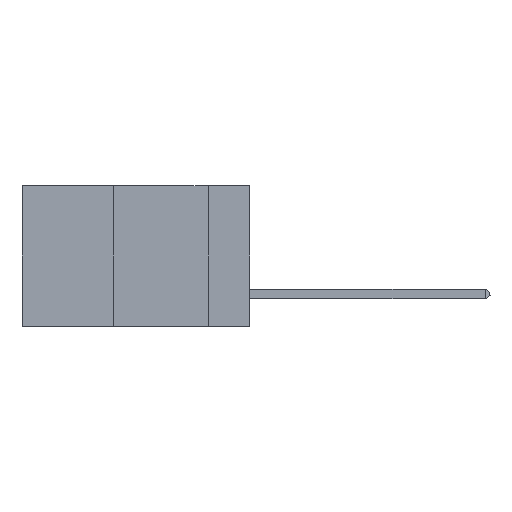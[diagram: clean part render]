
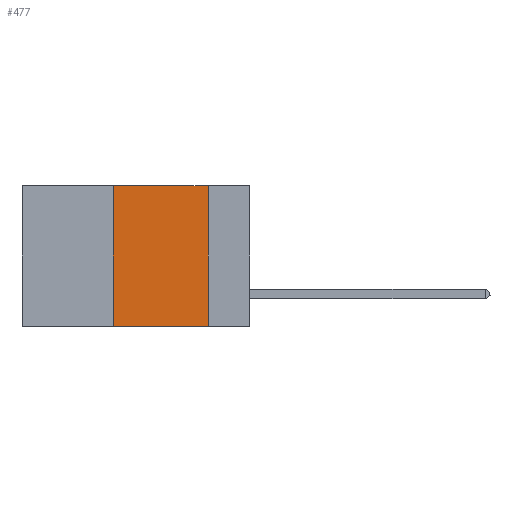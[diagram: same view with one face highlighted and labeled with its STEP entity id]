
A CAD part, left-side view. The second image highlights one B-rep face of the part: STEP entity #477.
In plain terms, the highlighted planar face has unit normal (-1, 0, 0).
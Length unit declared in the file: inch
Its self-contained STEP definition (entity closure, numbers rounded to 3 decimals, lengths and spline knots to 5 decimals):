
#151 = ORIENTED_EDGE ( 'NONE', *, *, #31321, .F. ) ;
#477 = ADVANCED_FACE ( 'NONE', ( #30734 ), #1263, .F. ) ;
#1263 = PLANE ( 'NONE',  #20618 ) ;
#2311 = LINE ( 'NONE', #8115, #15526 ) ;
#4240 = DIRECTION ( 'NONE',  ( 1., 0., 0. ) ) ;
#8035 = CARTESIAN_POINT ( 'NONE',  ( 0., 0.11, -0.37 ) ) ;
#8115 = CARTESIAN_POINT ( 'NONE',  ( 0., 0.36, 0. ) ) ;
#9543 = CARTESIAN_POINT ( 'NONE',  ( 0., 0.6, -0.37 ) ) ;
#12318 = CARTESIAN_POINT ( 'NONE',  ( 0., 0.6, 0. ) ) ;
#12811 = VERTEX_POINT ( 'NONE', #23126 ) ;
#14838 = LINE ( 'NONE', #23871, #15666 ) ;
#15526 = VECTOR ( 'NONE', #27342, 39.37008 ) ;
#15666 = VECTOR ( 'NONE', #31942, 39.37008 ) ;
#16629 = ORIENTED_EDGE ( 'NONE', *, *, #32675, .T. ) ;
#18580 = CARTESIAN_POINT ( 'NONE',  ( 0., 0.36, -0.37 ) ) ;
#20011 = EDGE_CURVE ( 'NONE', #21207, #20627, #14838, .T. ) ;
#20078 = CARTESIAN_POINT ( 'NONE',  ( 0., 0.6, 0. ) ) ;
#20618 = AXIS2_PLACEMENT_3D ( 'NONE', #12318, #4240, #30980 ) ;
#20627 = VERTEX_POINT ( 'NONE', #8035 ) ;
#21176 = DIRECTION ( 'NONE',  ( 0., -1., 0. ) ) ;
#21207 = VERTEX_POINT ( 'NONE', #27738 ) ;
#21573 = VECTOR ( 'NONE', #30868, 39.37008 ) ;
#22081 = EDGE_CURVE ( 'NONE', #12811, #21207, #25952, .T. ) ;
#23126 = CARTESIAN_POINT ( 'NONE',  ( 0., 0.36, 0. ) ) ;
#23871 = CARTESIAN_POINT ( 'NONE',  ( 0., 0.11, 0. ) ) ;
#25526 = VECTOR ( 'NONE', #21176, 39.37008 ) ;
#25952 = LINE ( 'NONE', #20078, #25526 ) ;
#27342 = DIRECTION ( 'NONE',  ( 0., 0., 1. ) ) ;
#27738 = CARTESIAN_POINT ( 'NONE',  ( 0., 0.11, 0. ) ) ;
#27911 = ORIENTED_EDGE ( 'NONE', *, *, #20011, .F. ) ;
#30734 = FACE_OUTER_BOUND ( 'NONE', #32633, .T. ) ;
#30868 = DIRECTION ( 'NONE',  ( 0., -1., 0. ) ) ;
#30980 = DIRECTION ( 'NONE',  ( 0., 0., -1. ) ) ;
#31321 = EDGE_CURVE ( 'NONE', #32310, #12811, #2311, .T. ) ;
#31942 = DIRECTION ( 'NONE',  ( 0., 0., -1. ) ) ;
#32218 = ORIENTED_EDGE ( 'NONE', *, *, #22081, .F. ) ;
#32310 = VERTEX_POINT ( 'NONE', #18580 ) ;
#32633 = EDGE_LOOP ( 'NONE', ( #27911, #32218, #151, #16629 ) ) ;
#32675 = EDGE_CURVE ( 'NONE', #32310, #20627, #32776, .T. ) ;
#32776 = LINE ( 'NONE', #9543, #21573 ) ;
